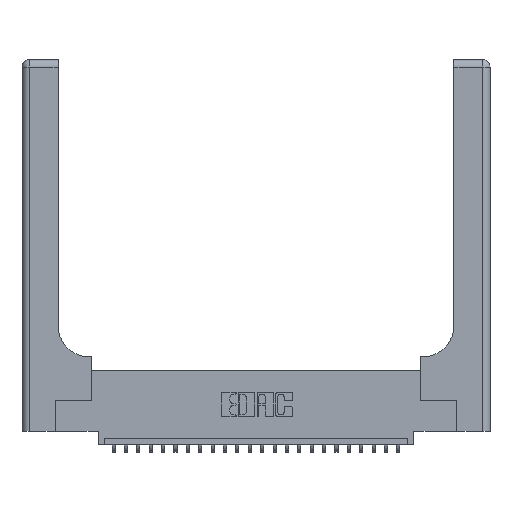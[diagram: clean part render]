
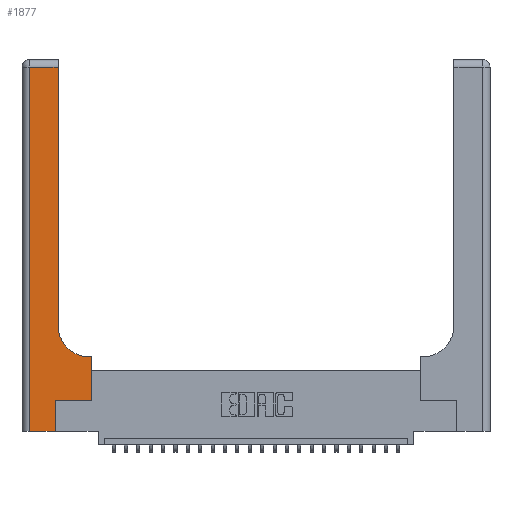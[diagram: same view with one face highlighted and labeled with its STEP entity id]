
A CAD part, top view. The second image highlights one B-rep face of the part: STEP entity #1877.
In plain terms, the highlighted planar face has unit normal (0, 0, 1).
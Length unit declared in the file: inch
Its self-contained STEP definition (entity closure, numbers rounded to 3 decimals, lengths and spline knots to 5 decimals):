
#100 = VECTOR ( 'NONE', #21575, 39.37008 ) ;
#154 = ORIENTED_EDGE ( 'NONE', *, *, #14048, .T. ) ;
#818 = CARTESIAN_POINT ( 'NONE',  ( 0.06, 2.94, 0.37 ) ) ;
#1381 = CARTESIAN_POINT ( 'NONE',  ( 0.06, 3., 0.37 ) ) ;
#1860 = DIRECTION ( 'NONE',  ( -1., 0., 0. ) ) ;
#1877 = ADVANCED_FACE ( 'NONE', ( #14276 ), #21559, .F. ) ;
#2395 = DIRECTION ( 'NONE',  ( 0., 0., -1. ) ) ;
#2752 = CARTESIAN_POINT ( 'NONE',  ( 0.5415, 0.6, 0.37 ) ) ;
#3015 = CARTESIAN_POINT ( 'NONE',  ( 0.269, 0., 0.37 ) ) ;
#3338 = VECTOR ( 'NONE', #5452, 39.37008 ) ;
#3811 = CARTESIAN_POINT ( 'NONE',  ( 0.269, 0.25, 0.37 ) ) ;
#4843 = DIRECTION ( 'NONE',  ( 0., 1., 0. ) ) ;
#5452 = DIRECTION ( 'NONE',  ( 0., 1., 0. ) ) ;
#5457 = LINE ( 'NONE', #1381, #100 ) ;
#5578 = DIRECTION ( 'NONE',  ( -1., 0., 0. ) ) ;
#5756 = VERTEX_POINT ( 'NONE', #12330 ) ;
#6548 = EDGE_CURVE ( 'NONE', #18941, #11825, #14906, .T. ) ;
#7111 = VECTOR ( 'NONE', #11411, 39.37008 ) ;
#7688 = VERTEX_POINT ( 'NONE', #818 ) ;
#7706 = VERTEX_POINT ( 'NONE', #2752 ) ;
#8213 = AXIS2_PLACEMENT_3D ( 'NONE', #18650, #2395, #24513 ) ;
#8583 = CIRCLE ( 'NONE', #8213, 0.25 ) ;
#9506 = CARTESIAN_POINT ( 'NONE',  ( 0., 0., 0.37 ) ) ;
#9511 = ORIENTED_EDGE ( 'NONE', *, *, #25797, .T. ) ;
#10217 = DIRECTION ( 'NONE',  ( -1., 0., 0. ) ) ;
#10351 = AXIS2_PLACEMENT_3D ( 'NONE', #15600, #11808, #1860 ) ;
#10642 = VECTOR ( 'NONE', #4843, 39.37008 ) ;
#11411 = DIRECTION ( 'NONE',  ( 1., 0., 0. ) ) ;
#11808 = DIRECTION ( 'NONE',  ( 0., 0., -1. ) ) ;
#11825 = VERTEX_POINT ( 'NONE', #17028 ) ;
#12330 = CARTESIAN_POINT ( 'NONE',  ( 0.2915, 2.94, 0.37 ) ) ;
#12395 = CARTESIAN_POINT ( 'NONE',  ( 0.2915, 0.6, 0.37 ) ) ;
#12488 = VERTEX_POINT ( 'NONE', #13953 ) ;
#12495 = ORIENTED_EDGE ( 'NONE', *, *, #6548, .T. ) ;
#12562 = CARTESIAN_POINT ( 'NONE',  ( 0.06, 0., 0.37 ) ) ;
#12689 = LINE ( 'NONE', #17621, #24282 ) ;
#13215 = VERTEX_POINT ( 'NONE', #23023 ) ;
#13953 = CARTESIAN_POINT ( 'NONE',  ( 0.5585, 0.6, 0.37 ) ) ;
#14048 = EDGE_CURVE ( 'NONE', #5756, #7688, #18638, .T. ) ;
#14276 = FACE_OUTER_BOUND ( 'NONE', #21152, .T. ) ;
#14286 = EDGE_CURVE ( 'NONE', #12488, #7706, #25816, .T. ) ;
#14717 = CARTESIAN_POINT ( 'NONE',  ( 0.5585, 0.25, 0.37 ) ) ;
#14906 = LINE ( 'NONE', #9506, #7111 ) ;
#15187 = LINE ( 'NONE', #25511, #3338 ) ;
#15401 = DIRECTION ( 'NONE',  ( 0., 1., 0. ) ) ;
#15515 = EDGE_CURVE ( 'NONE', #7706, #13215, #8583, .T. ) ;
#15600 = CARTESIAN_POINT ( 'NONE',  ( 0., 3., 0.37 ) ) ;
#16785 = LINE ( 'NONE', #3811, #23692 ) ;
#17028 = CARTESIAN_POINT ( 'NONE',  ( 0.269, 0., 0.37 ) ) ;
#17429 = VECTOR ( 'NONE', #10217, 39.37008 ) ;
#17432 = VERTEX_POINT ( 'NONE', #14717 ) ;
#17621 = CARTESIAN_POINT ( 'NONE',  ( 0.5585, 0.25, 0.37 ) ) ;
#17836 = ORIENTED_EDGE ( 'NONE', *, *, #21629, .T. ) ;
#18330 = CARTESIAN_POINT ( 'NONE',  ( 0.269, 0.25, 0.37 ) ) ;
#18484 = ORIENTED_EDGE ( 'NONE', *, *, #14286, .T. ) ;
#18638 = LINE ( 'NONE', #25219, #20534 ) ;
#18650 = CARTESIAN_POINT ( 'NONE',  ( 0.5415, 0.85, 0.37 ) ) ;
#18941 = VERTEX_POINT ( 'NONE', #12562 ) ;
#19139 = ORIENTED_EDGE ( 'NONE', *, *, #25623, .T. ) ;
#19196 = EDGE_CURVE ( 'NONE', #13215, #5756, #15187, .T. ) ;
#20534 = VECTOR ( 'NONE', #5578, 39.37008 ) ;
#21152 = EDGE_LOOP ( 'NONE', ( #22727, #154, #17836, #12495, #25702, #9511, #19139, #18484, #21381 ) ) ;
#21381 = ORIENTED_EDGE ( 'NONE', *, *, #15515, .T. ) ;
#21559 = PLANE ( 'NONE',  #10351 ) ;
#21575 = DIRECTION ( 'NONE',  ( 0., -1., 0. ) ) ;
#21629 = EDGE_CURVE ( 'NONE', #7688, #18941, #5457, .T. ) ;
#21984 = DIRECTION ( 'NONE',  ( 1., 0., 0. ) ) ;
#22260 = VERTEX_POINT ( 'NONE', #18330 ) ;
#22727 = ORIENTED_EDGE ( 'NONE', *, *, #19196, .T. ) ;
#23023 = CARTESIAN_POINT ( 'NONE',  ( 0.2915, 0.85, 0.37 ) ) ;
#23063 = EDGE_CURVE ( 'NONE', #11825, #22260, #24107, .T. ) ;
#23692 = VECTOR ( 'NONE', #21984, 39.37008 ) ;
#24107 = LINE ( 'NONE', #3015, #10642 ) ;
#24282 = VECTOR ( 'NONE', #15401, 39.37008 ) ;
#24513 = DIRECTION ( 'NONE',  ( 1., 0., 0. ) ) ;
#25219 = CARTESIAN_POINT ( 'NONE',  ( 0., 2.94, 0.37 ) ) ;
#25511 = CARTESIAN_POINT ( 'NONE',  ( 0.2915, 3., 0.37 ) ) ;
#25623 = EDGE_CURVE ( 'NONE', #17432, #12488, #12689, .T. ) ;
#25702 = ORIENTED_EDGE ( 'NONE', *, *, #23063, .T. ) ;
#25797 = EDGE_CURVE ( 'NONE', #22260, #17432, #16785, .T. ) ;
#25816 = LINE ( 'NONE', #12395, #17429 ) ;
